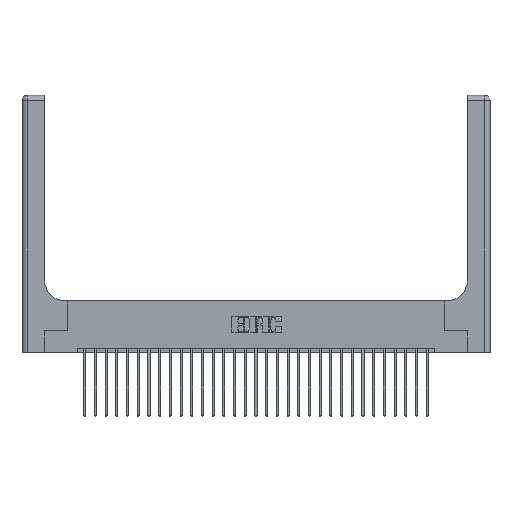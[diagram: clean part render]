
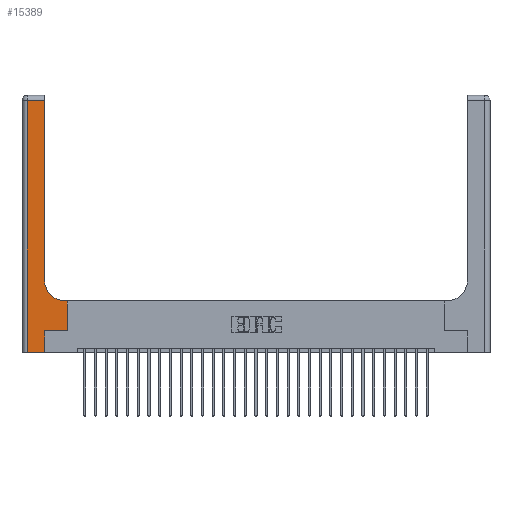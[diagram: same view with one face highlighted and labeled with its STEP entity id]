
A CAD part, top view. The second image highlights one B-rep face of the part: STEP entity #15389.
In plain terms, the highlighted planar face has unit normal (0, 0, 1).
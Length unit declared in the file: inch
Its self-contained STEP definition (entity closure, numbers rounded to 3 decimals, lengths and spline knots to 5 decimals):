
#507 = ORIENTED_EDGE ( 'NONE', *, *, #11335, .T. ) ;
#1025 = LINE ( 'NONE', #27333, #6715 ) ;
#1387 = VERTEX_POINT ( 'NONE', #5469 ) ;
#1541 = AXIS2_PLACEMENT_3D ( 'NONE', #17768, #6861, #13464 ) ;
#2121 = VECTOR ( 'NONE', #25452, 39.37008 ) ;
#2136 = VERTEX_POINT ( 'NONE', #9398 ) ;
#2358 = EDGE_CURVE ( 'NONE', #20808, #5355, #28201, .T. ) ;
#3719 = DIRECTION ( 'NONE',  ( 0., 0., -1. ) ) ;
#4199 = DIRECTION ( 'NONE',  ( -1., 0., 0. ) ) ;
#5128 = ORIENTED_EDGE ( 'NONE', *, *, #27679, .T. ) ;
#5355 = VERTEX_POINT ( 'NONE', #18749 ) ;
#5386 = ORIENTED_EDGE ( 'NONE', *, *, #7730, .T. ) ;
#5469 = CARTESIAN_POINT ( 'NONE',  ( 0.26, 0.85, 0.37 ) ) ;
#5784 = CARTESIAN_POINT ( 'NONE',  ( 0.265, 0., 0.37 ) ) ;
#5953 = EDGE_CURVE ( 'NONE', #21702, #2136, #28042, .T. ) ;
#6245 = VECTOR ( 'NONE', #21596, 39.37008 ) ;
#6715 = VECTOR ( 'NONE', #9655, 39.37008 ) ;
#6861 = DIRECTION ( 'NONE',  ( 0., 0., -1. ) ) ;
#7520 = VECTOR ( 'NONE', #24449, 39.37008 ) ;
#7730 = EDGE_CURVE ( 'NONE', #24825, #11789, #8081, .T. ) ;
#8081 = LINE ( 'NONE', #5784, #2121 ) ;
#8867 = PLANE ( 'NONE',  #1541 ) ;
#9122 = CARTESIAN_POINT ( 'NONE',  ( 0.26, 2.94, 0.37 ) ) ;
#9398 = CARTESIAN_POINT ( 'NONE',  ( 0.51, 0.6, 0.37 ) ) ;
#9584 = CARTESIAN_POINT ( 'NONE',  ( 0.265, 0.25, 0.37 ) ) ;
#9655 = DIRECTION ( 'NONE',  ( 0., 1., 0. ) ) ;
#10015 = LINE ( 'NONE', #20464, #16357 ) ;
#10672 = VERTEX_POINT ( 'NONE', #27959 ) ;
#10828 = CARTESIAN_POINT ( 'NONE',  ( 0.265, 0.25, 0.37 ) ) ;
#11173 = CARTESIAN_POINT ( 'NONE',  ( 0.528, 0.6, 0.37 ) ) ;
#11335 = EDGE_CURVE ( 'NONE', #2136, #1387, #22271, .T. ) ;
#11716 = EDGE_CURVE ( 'NONE', #10672, #24825, #10015, .T. ) ;
#11742 = VERTEX_POINT ( 'NONE', #12305 ) ;
#11789 = VERTEX_POINT ( 'NONE', #9584 ) ;
#12305 = CARTESIAN_POINT ( 'NONE',  ( 0.528, 0.25, 0.37 ) ) ;
#12515 = EDGE_CURVE ( 'NONE', #11742, #21702, #1025, .T. ) ;
#13464 = DIRECTION ( 'NONE',  ( -1., 0., 0. ) ) ;
#13969 = LINE ( 'NONE', #20268, #16314 ) ;
#15238 = CARTESIAN_POINT ( 'NONE',  ( 0., 2.94, 0.37 ) ) ;
#15389 = ADVANCED_FACE ( 'NONE', ( #21760 ), #8867, .F. ) ;
#15990 = DIRECTION ( 'NONE',  ( 1., 0., 0. ) ) ;
#15992 = ORIENTED_EDGE ( 'NONE', *, *, #11716, .T. ) ;
#16314 = VECTOR ( 'NONE', #18537, 39.37008 ) ;
#16357 = VECTOR ( 'NONE', #18318, 39.37008 ) ;
#16544 = ORIENTED_EDGE ( 'NONE', *, *, #12515, .T. ) ;
#16925 = CARTESIAN_POINT ( 'NONE',  ( 0.51, 0.85, 0.37 ) ) ;
#17135 = ORIENTED_EDGE ( 'NONE', *, *, #23723, .T. ) ;
#17768 = CARTESIAN_POINT ( 'NONE',  ( 0., 3., 0.37 ) ) ;
#18186 = ORIENTED_EDGE ( 'NONE', *, *, #27091, .T. ) ;
#18234 = VECTOR ( 'NONE', #19374, 39.37008 ) ;
#18318 = DIRECTION ( 'NONE',  ( 1., 0., 0. ) ) ;
#18537 = DIRECTION ( 'NONE',  ( 0., 1., 0. ) ) ;
#18749 = CARTESIAN_POINT ( 'NONE',  ( 0.06, 2.94, 0.37 ) ) ;
#19374 = DIRECTION ( 'NONE',  ( -1., 0., 0. ) ) ;
#19598 = LINE ( 'NONE', #22344, #6245 ) ;
#20268 = CARTESIAN_POINT ( 'NONE',  ( 0.26, 3., 0.37 ) ) ;
#20464 = CARTESIAN_POINT ( 'NONE',  ( 0., 0., 0.37 ) ) ;
#20808 = VERTEX_POINT ( 'NONE', #9122 ) ;
#21141 = ORIENTED_EDGE ( 'NONE', *, *, #2358, .T. ) ;
#21596 = DIRECTION ( 'NONE',  ( 0., -1., 0. ) ) ;
#21702 = VERTEX_POINT ( 'NONE', #11173 ) ;
#21760 = FACE_OUTER_BOUND ( 'NONE', #25250, .T. ) ;
#21843 = LINE ( 'NONE', #10828, #7520 ) ;
#22271 = CIRCLE ( 'NONE', #24598, 0.25 ) ;
#22344 = CARTESIAN_POINT ( 'NONE',  ( 0.06, 3., 0.37 ) ) ;
#22635 = CARTESIAN_POINT ( 'NONE',  ( 0.265, 0., 0.37 ) ) ;
#23103 = VECTOR ( 'NONE', #4199, 39.37008 ) ;
#23723 = EDGE_CURVE ( 'NONE', #11789, #11742, #21843, .T. ) ;
#24449 = DIRECTION ( 'NONE',  ( 1., 0., 0. ) ) ;
#24598 = AXIS2_PLACEMENT_3D ( 'NONE', #16925, #3719, #15990 ) ;
#24825 = VERTEX_POINT ( 'NONE', #22635 ) ;
#25250 = EDGE_LOOP ( 'NONE', ( #18186, #21141, #5128, #15992, #5386, #17135, #16544, #26851, #507 ) ) ;
#25452 = DIRECTION ( 'NONE',  ( 0., 1., 0. ) ) ;
#25863 = CARTESIAN_POINT ( 'NONE',  ( 0.26, 0.6, 0.37 ) ) ;
#26851 = ORIENTED_EDGE ( 'NONE', *, *, #5953, .T. ) ;
#27091 = EDGE_CURVE ( 'NONE', #1387, #20808, #13969, .T. ) ;
#27333 = CARTESIAN_POINT ( 'NONE',  ( 0.528, 0.25, 0.37 ) ) ;
#27679 = EDGE_CURVE ( 'NONE', #5355, #10672, #19598, .T. ) ;
#27959 = CARTESIAN_POINT ( 'NONE',  ( 0.06, 0., 0.37 ) ) ;
#28042 = LINE ( 'NONE', #25863, #18234 ) ;
#28201 = LINE ( 'NONE', #15238, #23103 ) ;
